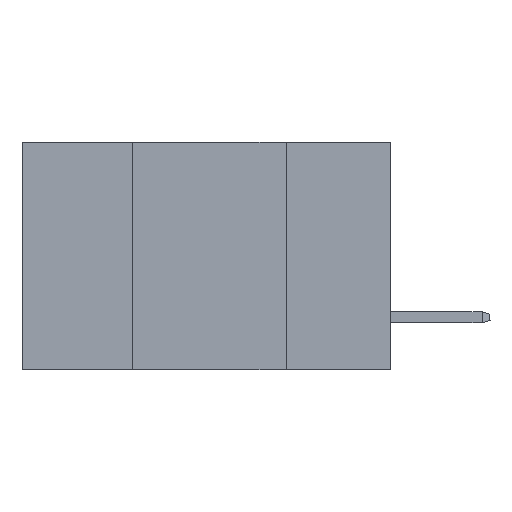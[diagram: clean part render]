
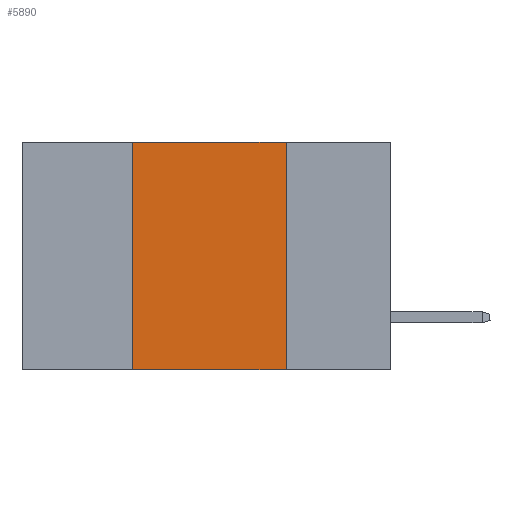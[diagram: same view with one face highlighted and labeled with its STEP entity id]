
A CAD part, left-side view. The second image highlights one B-rep face of the part: STEP entity #5890.
In plain terms, the highlighted planar face has unit normal (-1, 0, 0).
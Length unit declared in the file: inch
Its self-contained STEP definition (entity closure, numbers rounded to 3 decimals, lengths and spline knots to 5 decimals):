
#58 = VERTEX_POINT ( 'NONE', #11844 ) ;
#279 = VECTOR ( 'NONE', #2174, 39.37008 ) ;
#422 = VECTOR ( 'NONE', #11306, 39.37008 ) ;
#425 = LINE ( 'NONE', #4082, #279 ) ;
#830 = VERTEX_POINT ( 'NONE', #5412 ) ;
#921 = CARTESIAN_POINT ( 'NONE',  ( 0., 0.42, 0. ) ) ;
#1074 = ORIENTED_EDGE ( 'NONE', *, *, #1408, .F. ) ;
#1408 = EDGE_CURVE ( 'NONE', #3152, #58, #11248, .T. ) ;
#1571 = ORIENTED_EDGE ( 'NONE', *, *, #8478, .T. ) ;
#2081 = PLANE ( 'NONE',  #10722 ) ;
#2174 = DIRECTION ( 'NONE',  ( 0., 0., 1. ) ) ;
#2283 = EDGE_CURVE ( 'NONE', #58, #830, #4339, .T. ) ;
#2703 = DIRECTION ( 'NONE',  ( 1., 0., 0. ) ) ;
#3152 = VERTEX_POINT ( 'NONE', #921 ) ;
#3367 = VECTOR ( 'NONE', #5521, 39.37008 ) ;
#3851 = CARTESIAN_POINT ( 'NONE',  ( 0., 0.6, 0. ) ) ;
#4082 = CARTESIAN_POINT ( 'NONE',  ( 0., 0.42, 0. ) ) ;
#4339 = LINE ( 'NONE', #6121, #6223 ) ;
#5157 = EDGE_CURVE ( 'NONE', #5893, #3152, #425, .T. ) ;
#5212 = FACE_OUTER_BOUND ( 'NONE', #6230, .T. ) ;
#5412 = CARTESIAN_POINT ( 'NONE',  ( 0., 0.17, -0.37 ) ) ;
#5464 = ORIENTED_EDGE ( 'NONE', *, *, #5157, .F. ) ;
#5521 = DIRECTION ( 'NONE',  ( 0., -1., 0. ) ) ;
#5890 = ADVANCED_FACE ( 'NONE', ( #5212 ), #2081, .F. ) ;
#5893 = VERTEX_POINT ( 'NONE', #9479 ) ;
#6121 = CARTESIAN_POINT ( 'NONE',  ( 0., 0.17, 0. ) ) ;
#6223 = VECTOR ( 'NONE', #7962, 39.37008 ) ;
#6230 = EDGE_LOOP ( 'NONE', ( #10535, #1074, #5464, #1571 ) ) ;
#7962 = DIRECTION ( 'NONE',  ( 0., 0., -1. ) ) ;
#8218 = LINE ( 'NONE', #9223, #3367 ) ;
#8478 = EDGE_CURVE ( 'NONE', #5893, #830, #8218, .T. ) ;
#8641 = CARTESIAN_POINT ( 'NONE',  ( 0., 0.6, 0. ) ) ;
#9223 = CARTESIAN_POINT ( 'NONE',  ( 0., 0.6, -0.37 ) ) ;
#9479 = CARTESIAN_POINT ( 'NONE',  ( 0., 0.42, -0.37 ) ) ;
#10039 = DIRECTION ( 'NONE',  ( 0., 0., -1. ) ) ;
#10535 = ORIENTED_EDGE ( 'NONE', *, *, #2283, .F. ) ;
#10722 = AXIS2_PLACEMENT_3D ( 'NONE', #8641, #2703, #10039 ) ;
#11248 = LINE ( 'NONE', #3851, #422 ) ;
#11306 = DIRECTION ( 'NONE',  ( 0., -1., 0. ) ) ;
#11844 = CARTESIAN_POINT ( 'NONE',  ( 0., 0.17, 0. ) ) ;
